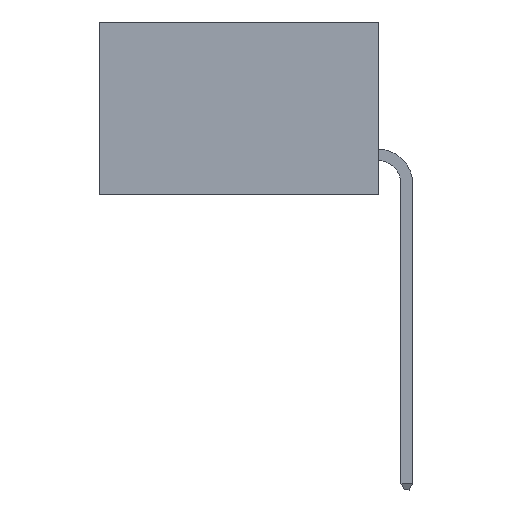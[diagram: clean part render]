
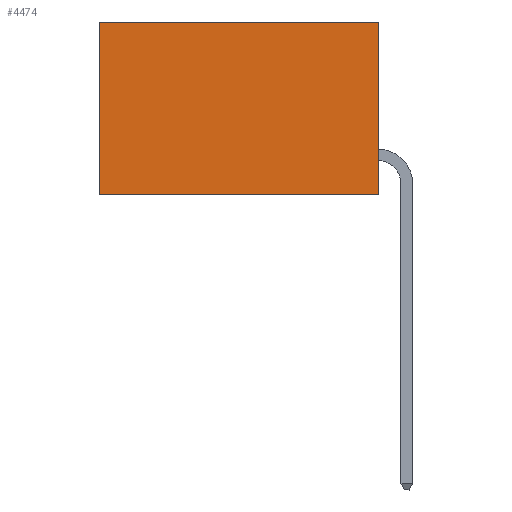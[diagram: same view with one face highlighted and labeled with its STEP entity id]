
A CAD part, left-side view. The second image highlights one B-rep face of the part: STEP entity #4474.
In plain terms, the highlighted planar face has unit normal (-1, 0, 0).
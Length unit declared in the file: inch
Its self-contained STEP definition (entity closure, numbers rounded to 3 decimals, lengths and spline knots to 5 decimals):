
#179 = DIRECTION ( 'NONE',  ( 0., 0., -1. ) ) ;
#292 = CARTESIAN_POINT ( 'NONE',  ( 0.2615, 0.6, 0. ) ) ;
#503 = EDGE_CURVE ( 'NONE', #5370, #4204, #8840, .T. ) ;
#763 = CARTESIAN_POINT ( 'NONE',  ( 0.2615, 0., -0.37 ) ) ;
#1002 = ORIENTED_EDGE ( 'NONE', *, *, #8025, .F. ) ;
#1241 = ORIENTED_EDGE ( 'NONE', *, *, #7894, .T. ) ;
#1407 = VECTOR ( 'NONE', #7848, 39.37008 ) ;
#2289 = EDGE_LOOP ( 'NONE', ( #5345, #1002, #7200, #1241 ) ) ;
#2413 = AXIS2_PLACEMENT_3D ( 'NONE', #7709, #3989, #179 ) ;
#2504 = PLANE ( 'NONE',  #2413 ) ;
#2855 = VERTEX_POINT ( 'NONE', #292 ) ;
#3311 = LINE ( 'NONE', #6277, #1407 ) ;
#3439 = VERTEX_POINT ( 'NONE', #6115 ) ;
#3741 = VECTOR ( 'NONE', #7653, 39.37008 ) ;
#3989 = DIRECTION ( 'NONE',  ( 1., 0., 0. ) ) ;
#4143 = CARTESIAN_POINT ( 'NONE',  ( 0.2615, 0., -0.37 ) ) ;
#4204 = VERTEX_POINT ( 'NONE', #6636 ) ;
#4468 = VECTOR ( 'NONE', #5806, 39.37008 ) ;
#4474 = ADVANCED_FACE ( 'NONE', ( #6183 ), #2504, .F. ) ;
#4967 = DIRECTION ( 'NONE',  ( 0., 1., 0. ) ) ;
#5345 = ORIENTED_EDGE ( 'NONE', *, *, #6732, .T. ) ;
#5370 = VERTEX_POINT ( 'NONE', #6944 ) ;
#5806 = DIRECTION ( 'NONE',  ( 0., 0., -1. ) ) ;
#6115 = CARTESIAN_POINT ( 'NONE',  ( 0.2615, 0.6, -0.37 ) ) ;
#6183 = FACE_OUTER_BOUND ( 'NONE', #2289, .T. ) ;
#6277 = CARTESIAN_POINT ( 'NONE',  ( 0.2615, 0.6, -0.37 ) ) ;
#6636 = CARTESIAN_POINT ( 'NONE',  ( 0.2615, 0., -0.37 ) ) ;
#6732 = EDGE_CURVE ( 'NONE', #2855, #3439, #3311, .T. ) ;
#6944 = CARTESIAN_POINT ( 'NONE',  ( 0.2615, 0., 0. ) ) ;
#7200 = ORIENTED_EDGE ( 'NONE', *, *, #503, .F. ) ;
#7465 = VECTOR ( 'NONE', #4967, 39.37008 ) ;
#7653 = DIRECTION ( 'NONE',  ( 0., 1., 0. ) ) ;
#7709 = CARTESIAN_POINT ( 'NONE',  ( 0.2615, 0., -0.37 ) ) ;
#7848 = DIRECTION ( 'NONE',  ( 0., 0., -1. ) ) ;
#7862 = LINE ( 'NONE', #4143, #7465 ) ;
#7894 = EDGE_CURVE ( 'NONE', #5370, #2855, #9094, .T. ) ;
#8025 = EDGE_CURVE ( 'NONE', #4204, #3439, #7862, .T. ) ;
#8840 = LINE ( 'NONE', #763, #4468 ) ;
#9094 = LINE ( 'NONE', #9280, #3741 ) ;
#9280 = CARTESIAN_POINT ( 'NONE',  ( 0.2615, 0., 0. ) ) ;
